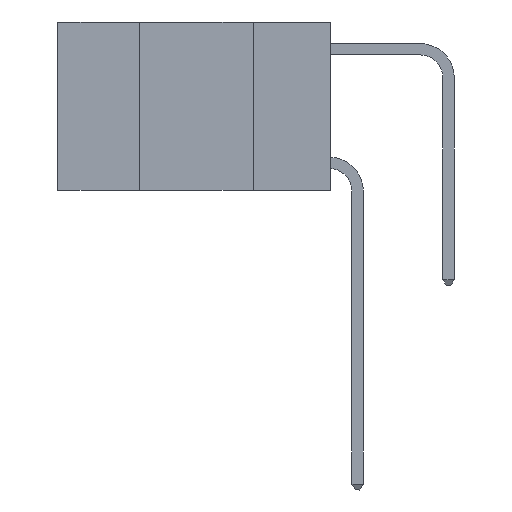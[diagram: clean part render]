
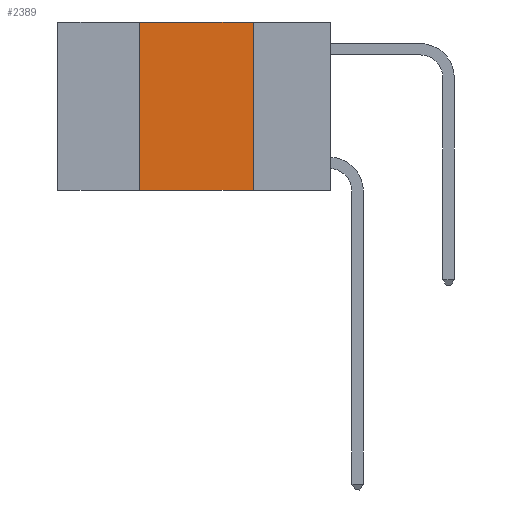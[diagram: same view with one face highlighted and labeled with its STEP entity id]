
A CAD part, left-side view. The second image highlights one B-rep face of the part: STEP entity #2389.
In plain terms, the highlighted planar face has unit normal (-1, 0, 0).
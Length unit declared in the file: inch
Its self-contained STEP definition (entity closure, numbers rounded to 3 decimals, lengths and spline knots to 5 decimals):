
#1258 = PLANE ( 'NONE',  #8783 ) ;
#2080 = DIRECTION ( 'NONE',  ( 1., 0., 0. ) ) ;
#2251 = DIRECTION ( 'NONE',  ( 0., 0., -1. ) ) ;
#2278 = CARTESIAN_POINT ( 'NONE',  ( 0., 0.17, 0. ) ) ;
#2389 = ADVANCED_FACE ( 'NONE', ( #11218 ), #1258, .F. ) ;
#2542 = VERTEX_POINT ( 'NONE', #12407 ) ;
#2792 = ORIENTED_EDGE ( 'NONE', *, *, #4479, .F. ) ;
#3377 = CARTESIAN_POINT ( 'NONE',  ( 0., 0.6, -0.37 ) ) ;
#3613 = CARTESIAN_POINT ( 'NONE',  ( 0., 0.42, -0.37 ) ) ;
#4003 = VERTEX_POINT ( 'NONE', #2278 ) ;
#4157 = CARTESIAN_POINT ( 'NONE',  ( 0., 0.6, 0. ) ) ;
#4479 = EDGE_CURVE ( 'NONE', #2542, #4003, #8500, .T. ) ;
#5015 = CARTESIAN_POINT ( 'NONE',  ( 0., 0.42, 0. ) ) ;
#5435 = EDGE_CURVE ( 'NONE', #7773, #13178, #9613, .T. ) ;
#6273 = DIRECTION ( 'NONE',  ( 0., 0., -1. ) ) ;
#6450 = DIRECTION ( 'NONE',  ( 0., -1., 0. ) ) ;
#6905 = EDGE_LOOP ( 'NONE', ( #7933, #2792, #7998, #10790 ) ) ;
#7107 = VECTOR ( 'NONE', #6450, 39.37008 ) ;
#7300 = VECTOR ( 'NONE', #7360, 39.37008 ) ;
#7360 = DIRECTION ( 'NONE',  ( 0., -1., 0. ) ) ;
#7579 = CARTESIAN_POINT ( 'NONE',  ( 0., 0.6, 0. ) ) ;
#7695 = VECTOR ( 'NONE', #2251, 39.37008 ) ;
#7773 = VERTEX_POINT ( 'NONE', #3613 ) ;
#7933 = ORIENTED_EDGE ( 'NONE', *, *, #10113, .F. ) ;
#7998 = ORIENTED_EDGE ( 'NONE', *, *, #10798, .F. ) ;
#8490 = LINE ( 'NONE', #10455, #7695 ) ;
#8500 = LINE ( 'NONE', #7579, #7107 ) ;
#8783 = AXIS2_PLACEMENT_3D ( 'NONE', #4157, #2080, #6273 ) ;
#8934 = DIRECTION ( 'NONE',  ( 0., 0., 1. ) ) ;
#9613 = LINE ( 'NONE', #3377, #7300 ) ;
#10113 = EDGE_CURVE ( 'NONE', #4003, #13178, #8490, .T. ) ;
#10158 = LINE ( 'NONE', #5015, #13034 ) ;
#10455 = CARTESIAN_POINT ( 'NONE',  ( 0., 0.17, 0. ) ) ;
#10790 = ORIENTED_EDGE ( 'NONE', *, *, #5435, .T. ) ;
#10798 = EDGE_CURVE ( 'NONE', #7773, #2542, #10158, .T. ) ;
#11218 = FACE_OUTER_BOUND ( 'NONE', #6905, .T. ) ;
#12407 = CARTESIAN_POINT ( 'NONE',  ( 0., 0.42, 0. ) ) ;
#12783 = CARTESIAN_POINT ( 'NONE',  ( 0., 0.17, -0.37 ) ) ;
#13034 = VECTOR ( 'NONE', #8934, 39.37008 ) ;
#13178 = VERTEX_POINT ( 'NONE', #12783 ) ;
